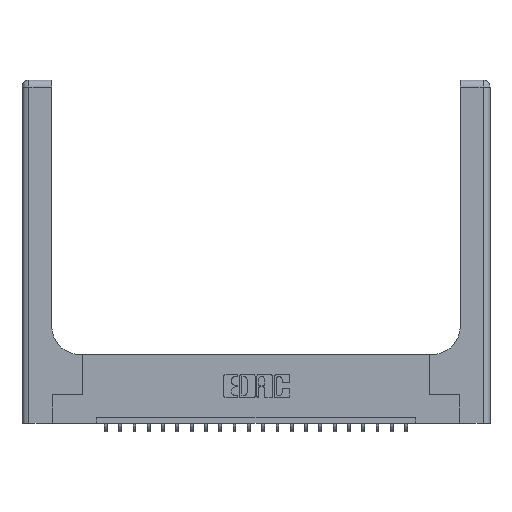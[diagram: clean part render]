
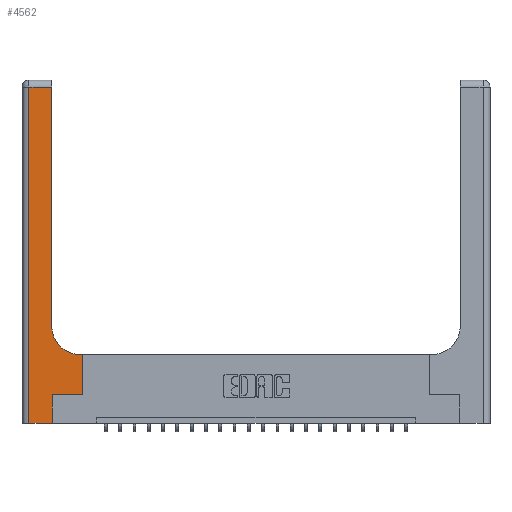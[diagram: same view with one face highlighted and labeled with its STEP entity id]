
A CAD part, top view. The second image highlights one B-rep face of the part: STEP entity #4562.
In plain terms, the highlighted planar face has unit normal (0, 0, 1).
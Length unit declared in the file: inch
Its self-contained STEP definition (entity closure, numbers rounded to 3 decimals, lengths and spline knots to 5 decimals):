
#98 = VECTOR ( 'NONE', #19377, 39.37008 ) ;
#539 = CARTESIAN_POINT ( 'NONE',  ( 0.265, 0.25, 0.37 ) ) ;
#1765 = EDGE_CURVE ( 'NONE', #5858, #18378, #20051, .T. ) ;
#1938 = EDGE_CURVE ( 'NONE', #13776, #9451, #19295, .T. ) ;
#1990 = CARTESIAN_POINT ( 'NONE',  ( 0.06, 0., 0.37 ) ) ;
#2012 = DIRECTION ( 'NONE',  ( -1., 0., 0. ) ) ;
#2325 = CARTESIAN_POINT ( 'NONE',  ( 0.528, 0.6, 0.37 ) ) ;
#2327 = CARTESIAN_POINT ( 'NONE',  ( 0.26, 3., 0.37 ) ) ;
#2446 = CARTESIAN_POINT ( 'NONE',  ( 0.26, 0.6, 0.37 ) ) ;
#3285 = AXIS2_PLACEMENT_3D ( 'NONE', #19524, #4245, #2012 ) ;
#3732 = LINE ( 'NONE', #3956, #20254 ) ;
#3895 = LINE ( 'NONE', #539, #98 ) ;
#3942 = EDGE_CURVE ( 'NONE', #21761, #13739, #16871, .T. ) ;
#3956 = CARTESIAN_POINT ( 'NONE',  ( 0., 0., 0.37 ) ) ;
#4245 = DIRECTION ( 'NONE',  ( 0., 0., -1. ) ) ;
#4562 = ADVANCED_FACE ( 'NONE', ( #12702 ), #11049, .F. ) ;
#4936 = EDGE_CURVE ( 'NONE', #18378, #21761, #3895, .T. ) ;
#4985 = VECTOR ( 'NONE', #9366, 39.37008 ) ;
#5287 = ORIENTED_EDGE ( 'NONE', *, *, #3942, .T. ) ;
#5759 = AXIS2_PLACEMENT_3D ( 'NONE', #15232, #18583, #6790 ) ;
#5858 = VERTEX_POINT ( 'NONE', #9607 ) ;
#6077 = CARTESIAN_POINT ( 'NONE',  ( 0.26, 0.85, 0.37 ) ) ;
#6246 = VECTOR ( 'NONE', #20362, 39.37008 ) ;
#6778 = VERTEX_POINT ( 'NONE', #9491 ) ;
#6790 = DIRECTION ( 'NONE',  ( 1., 0., 0. ) ) ;
#6814 = VECTOR ( 'NONE', #21840, 39.37008 ) ;
#6820 = LINE ( 'NONE', #8488, #16918 ) ;
#6854 = ORIENTED_EDGE ( 'NONE', *, *, #8256, .T. ) ;
#7089 = VERTEX_POINT ( 'NONE', #1990 ) ;
#7241 = ORIENTED_EDGE ( 'NONE', *, *, #15031, .T. ) ;
#7665 = CARTESIAN_POINT ( 'NONE',  ( 0.528, 0.25, 0.37 ) ) ;
#7986 = DIRECTION ( 'NONE',  ( 0., -1., 0. ) ) ;
#8256 = EDGE_CURVE ( 'NONE', #6778, #20304, #6820, .T. ) ;
#8488 = CARTESIAN_POINT ( 'NONE',  ( 0., 2.94, 0.37 ) ) ;
#8757 = VECTOR ( 'NONE', #14470, 39.37008 ) ;
#9366 = DIRECTION ( 'NONE',  ( -1., 0., 0. ) ) ;
#9451 = VERTEX_POINT ( 'NONE', #6077 ) ;
#9491 = CARTESIAN_POINT ( 'NONE',  ( 0.26, 2.94, 0.37 ) ) ;
#9607 = CARTESIAN_POINT ( 'NONE',  ( 0.265, 0., 0.37 ) ) ;
#10382 = ORIENTED_EDGE ( 'NONE', *, *, #4936, .T. ) ;
#10838 = ORIENTED_EDGE ( 'NONE', *, *, #20981, .T. ) ;
#11049 = PLANE ( 'NONE',  #3285 ) ;
#11197 = EDGE_LOOP ( 'NONE', ( #11987, #6854, #15307, #10838, #18551, #10382, #5287, #7241, #12993 ) ) ;
#11562 = CARTESIAN_POINT ( 'NONE',  ( 0.265, 0., 0.37 ) ) ;
#11987 = ORIENTED_EDGE ( 'NONE', *, *, #18225, .T. ) ;
#12626 = DIRECTION ( 'NONE',  ( 1., 0., 0. ) ) ;
#12702 = FACE_OUTER_BOUND ( 'NONE', #11197, .T. ) ;
#12704 = EDGE_CURVE ( 'NONE', #20304, #7089, #21820, .T. ) ;
#12993 = ORIENTED_EDGE ( 'NONE', *, *, #1938, .T. ) ;
#13424 = CARTESIAN_POINT ( 'NONE',  ( 0.06, 3., 0.37 ) ) ;
#13458 = CARTESIAN_POINT ( 'NONE',  ( 0.265, 0.25, 0.37 ) ) ;
#13739 = VERTEX_POINT ( 'NONE', #2325 ) ;
#13776 = VERTEX_POINT ( 'NONE', #14142 ) ;
#14142 = CARTESIAN_POINT ( 'NONE',  ( 0.51, 0.6, 0.37 ) ) ;
#14470 = DIRECTION ( 'NONE',  ( 0., 1., 0. ) ) ;
#15031 = EDGE_CURVE ( 'NONE', #13739, #13776, #19186, .T. ) ;
#15232 = CARTESIAN_POINT ( 'NONE',  ( 0.51, 0.85, 0.37 ) ) ;
#15307 = ORIENTED_EDGE ( 'NONE', *, *, #12704, .T. ) ;
#16871 = LINE ( 'NONE', #20580, #6246 ) ;
#16918 = VECTOR ( 'NONE', #20855, 39.37008 ) ;
#17597 = LINE ( 'NONE', #2327, #8757 ) ;
#18225 = EDGE_CURVE ( 'NONE', #9451, #6778, #17597, .T. ) ;
#18378 = VERTEX_POINT ( 'NONE', #13458 ) ;
#18551 = ORIENTED_EDGE ( 'NONE', *, *, #1765, .T. ) ;
#18583 = DIRECTION ( 'NONE',  ( 0., 0., -1. ) ) ;
#19166 = VECTOR ( 'NONE', #7986, 39.37008 ) ;
#19186 = LINE ( 'NONE', #2446, #4985 ) ;
#19295 = CIRCLE ( 'NONE', #5759, 0.25 ) ;
#19377 = DIRECTION ( 'NONE',  ( 1., 0., 0. ) ) ;
#19524 = CARTESIAN_POINT ( 'NONE',  ( 0., 3., 0.37 ) ) ;
#20051 = LINE ( 'NONE', #11562, #6814 ) ;
#20254 = VECTOR ( 'NONE', #12626, 39.37008 ) ;
#20304 = VERTEX_POINT ( 'NONE', #21734 ) ;
#20362 = DIRECTION ( 'NONE',  ( 0., 1., 0. ) ) ;
#20580 = CARTESIAN_POINT ( 'NONE',  ( 0.528, 0.25, 0.37 ) ) ;
#20855 = DIRECTION ( 'NONE',  ( -1., 0., 0. ) ) ;
#20981 = EDGE_CURVE ( 'NONE', #7089, #5858, #3732, .T. ) ;
#21734 = CARTESIAN_POINT ( 'NONE',  ( 0.06, 2.94, 0.37 ) ) ;
#21761 = VERTEX_POINT ( 'NONE', #7665 ) ;
#21820 = LINE ( 'NONE', #13424, #19166 ) ;
#21840 = DIRECTION ( 'NONE',  ( 0., 1., 0. ) ) ;
